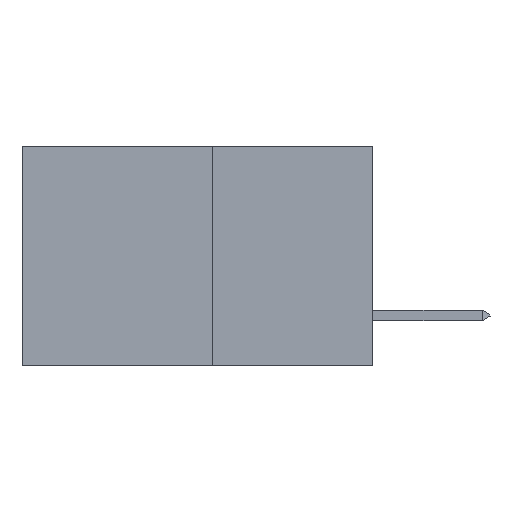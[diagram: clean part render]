
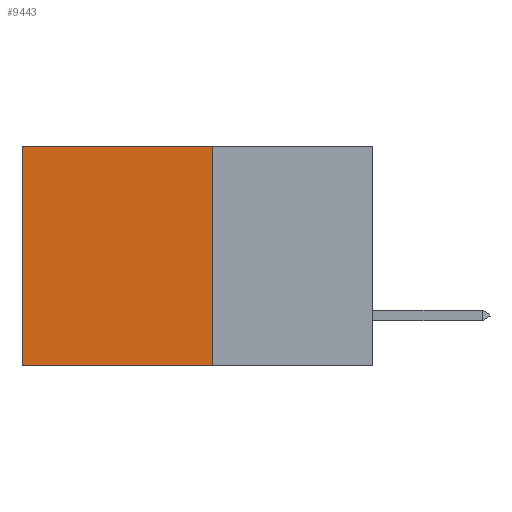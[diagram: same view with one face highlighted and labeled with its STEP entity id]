
A CAD part, left-side view. The second image highlights one B-rep face of the part: STEP entity #9443.
In plain terms, the highlighted planar face has unit normal (-1, 0, 0).
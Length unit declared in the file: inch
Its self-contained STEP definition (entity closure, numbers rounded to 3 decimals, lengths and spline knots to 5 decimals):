
#1110 = CARTESIAN_POINT ( 'NONE',  ( 0.277, 0.27, -0.37 ) ) ;
#1938 = AXIS2_PLACEMENT_3D ( 'NONE', #5302, #18112, #3378 ) ;
#2292 = CARTESIAN_POINT ( 'NONE',  ( 0.277, 0.27, 0. ) ) ;
#3347 = DIRECTION ( 'NONE',  ( 0., 0., -1. ) ) ;
#3378 = DIRECTION ( 'NONE',  ( 0., 0., -1. ) ) ;
#3696 = EDGE_CURVE ( 'NONE', #5220, #22975, #10014, .T. ) ;
#3848 = CARTESIAN_POINT ( 'NONE',  ( 0.277, 0.59, -0.37 ) ) ;
#4885 = CARTESIAN_POINT ( 'NONE',  ( 0.277, 0.27, -0.37 ) ) ;
#5220 = VERTEX_POINT ( 'NONE', #6715 ) ;
#5302 = CARTESIAN_POINT ( 'NONE',  ( 0.277, 0.27, -0.37 ) ) ;
#5703 = FACE_OUTER_BOUND ( 'NONE', #9186, .T. ) ;
#6715 = CARTESIAN_POINT ( 'NONE',  ( 0.277, 0.59, 0. ) ) ;
#9007 = VECTOR ( 'NONE', #26812, 39.37008 ) ;
#9186 = EDGE_LOOP ( 'NONE', ( #16971, #30355, #25866, #13935 ) ) ;
#9443 = ADVANCED_FACE ( 'NONE', ( #5703 ), #11593, .F. ) ;
#9785 = LINE ( 'NONE', #4885, #9007 ) ;
#9938 = VECTOR ( 'NONE', #30329, 39.37008 ) ;
#10014 = LINE ( 'NONE', #3848, #22191 ) ;
#11593 = PLANE ( 'NONE',  #1938 ) ;
#12009 = DIRECTION ( 'NONE',  ( 0., 1., 0. ) ) ;
#12956 = LINE ( 'NONE', #2292, #18624 ) ;
#13935 = ORIENTED_EDGE ( 'NONE', *, *, #25288, .T. ) ;
#13945 = CARTESIAN_POINT ( 'NONE',  ( 0.277, 0.27, -0.37 ) ) ;
#16971 = ORIENTED_EDGE ( 'NONE', *, *, #3696, .T. ) ;
#17092 = EDGE_CURVE ( 'NONE', #23289, #22975, #29354, .T. ) ;
#17098 = VERTEX_POINT ( 'NONE', #18200 ) ;
#18112 = DIRECTION ( 'NONE',  ( 1., 0., 0. ) ) ;
#18200 = CARTESIAN_POINT ( 'NONE',  ( 0.277, 0.27, 0. ) ) ;
#18624 = VECTOR ( 'NONE', #12009, 39.37008 ) ;
#19328 = EDGE_CURVE ( 'NONE', #17098, #23289, #9785, .T. ) ;
#19965 = CARTESIAN_POINT ( 'NONE',  ( 0.277, 0.59, -0.37 ) ) ;
#22191 = VECTOR ( 'NONE', #3347, 39.37008 ) ;
#22975 = VERTEX_POINT ( 'NONE', #19965 ) ;
#23289 = VERTEX_POINT ( 'NONE', #13945 ) ;
#25288 = EDGE_CURVE ( 'NONE', #17098, #5220, #12956, .T. ) ;
#25866 = ORIENTED_EDGE ( 'NONE', *, *, #19328, .F. ) ;
#26812 = DIRECTION ( 'NONE',  ( 0., 0., -1. ) ) ;
#29354 = LINE ( 'NONE', #1110, #9938 ) ;
#30329 = DIRECTION ( 'NONE',  ( 0., 1., 0. ) ) ;
#30355 = ORIENTED_EDGE ( 'NONE', *, *, #17092, .F. ) ;
